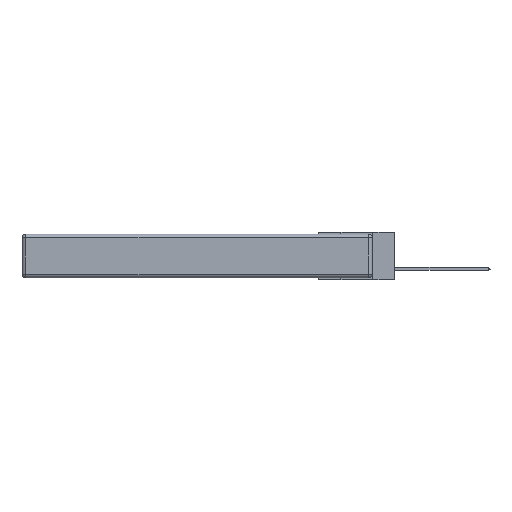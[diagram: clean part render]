
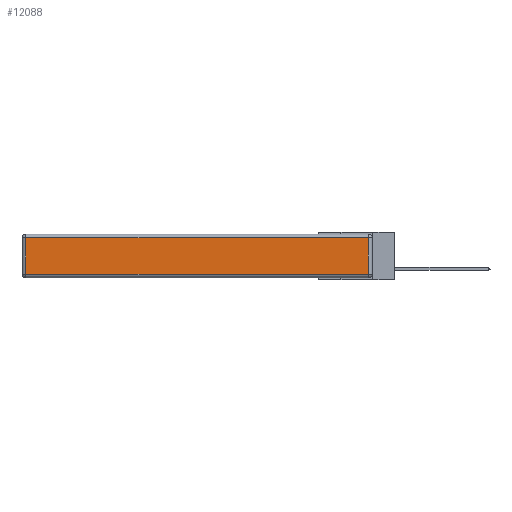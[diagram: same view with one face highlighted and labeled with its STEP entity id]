
A CAD part, left-side view. The second image highlights one B-rep face of the part: STEP entity #12088.
In plain terms, the highlighted planar face has unit normal (-1, 0, 0).
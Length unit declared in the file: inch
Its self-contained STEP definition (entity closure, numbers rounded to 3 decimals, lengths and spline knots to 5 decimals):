
#321 = DIRECTION ( 'NONE',  ( 0., 0., 1. ) ) ;
#455 = LINE ( 'NONE', #1697, #4469 ) ;
#1126 = CARTESIAN_POINT ( 'NONE',  ( 0., 2.72, -0.313 ) ) ;
#1362 = VERTEX_POINT ( 'NONE', #12225 ) ;
#1638 = CARTESIAN_POINT ( 'NONE',  ( 0., 0., -0.343 ) ) ;
#1697 = CARTESIAN_POINT ( 'NONE',  ( 0., 2.72, -0.343 ) ) ;
#1705 = DIRECTION ( 'NONE',  ( 0., 1., 0. ) ) ;
#1841 = EDGE_CURVE ( 'NONE', #11859, #10422, #455, .T. ) ;
#2372 = EDGE_CURVE ( 'NONE', #10422, #8624, #5013, .T. ) ;
#2549 = DIRECTION ( 'NONE',  ( -1., 0., 0. ) ) ;
#3223 = AXIS2_PLACEMENT_3D ( 'NONE', #1638, #2549, #321 ) ;
#3244 = CARTESIAN_POINT ( 'NONE',  ( 0., 0.03, -0.313 ) ) ;
#3667 = ORIENTED_EDGE ( 'NONE', *, *, #1841, .T. ) ;
#3788 = DIRECTION ( 'NONE',  ( 0., 0., -1. ) ) ;
#4206 = DIRECTION ( 'NONE',  ( 0., 0., 1. ) ) ;
#4288 = VECTOR ( 'NONE', #12803, 39.37008 ) ;
#4290 = LINE ( 'NONE', #7696, #6931 ) ;
#4436 = EDGE_LOOP ( 'NONE', ( #10459, #10070, #12103, #3667 ) ) ;
#4469 = VECTOR ( 'NONE', #3788, 39.37008 ) ;
#4635 = LINE ( 'NONE', #8410, #12828 ) ;
#4909 = CARTESIAN_POINT ( 'NONE',  ( 0., 0., -0.313 ) ) ;
#5013 = LINE ( 'NONE', #4909, #4288 ) ;
#6931 = VECTOR ( 'NONE', #4206, 39.37008 ) ;
#7672 = CARTESIAN_POINT ( 'NONE',  ( 0., 2.72, -0.03 ) ) ;
#7696 = CARTESIAN_POINT ( 'NONE',  ( 0., 0.03, -0.343 ) ) ;
#8410 = CARTESIAN_POINT ( 'NONE',  ( 0., 2.75, -0.03 ) ) ;
#8624 = VERTEX_POINT ( 'NONE', #3244 ) ;
#9269 = PLANE ( 'NONE',  #3223 ) ;
#9384 = FACE_OUTER_BOUND ( 'NONE', #4436, .T. ) ;
#9569 = EDGE_CURVE ( 'NONE', #8624, #1362, #4290, .T. ) ;
#10070 = ORIENTED_EDGE ( 'NONE', *, *, #9569, .T. ) ;
#10422 = VERTEX_POINT ( 'NONE', #1126 ) ;
#10459 = ORIENTED_EDGE ( 'NONE', *, *, #2372, .T. ) ;
#10658 = EDGE_CURVE ( 'NONE', #1362, #11859, #4635, .T. ) ;
#11859 = VERTEX_POINT ( 'NONE', #7672 ) ;
#12088 = ADVANCED_FACE ( 'NONE', ( #9384 ), #9269, .T. ) ;
#12103 = ORIENTED_EDGE ( 'NONE', *, *, #10658, .T. ) ;
#12225 = CARTESIAN_POINT ( 'NONE',  ( 0., 0.03, -0.03 ) ) ;
#12803 = DIRECTION ( 'NONE',  ( 0., -1., 0. ) ) ;
#12828 = VECTOR ( 'NONE', #1705, 39.37008 ) ;
